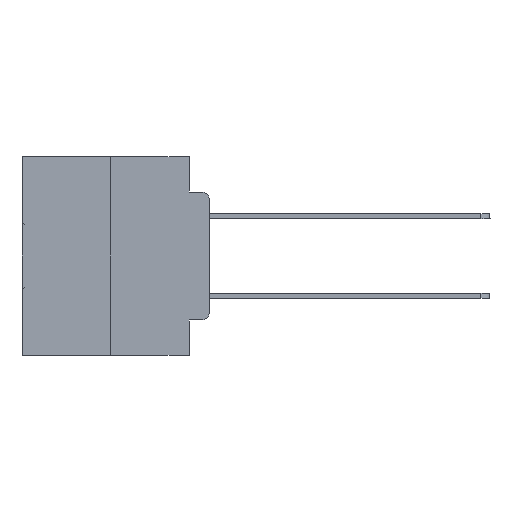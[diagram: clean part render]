
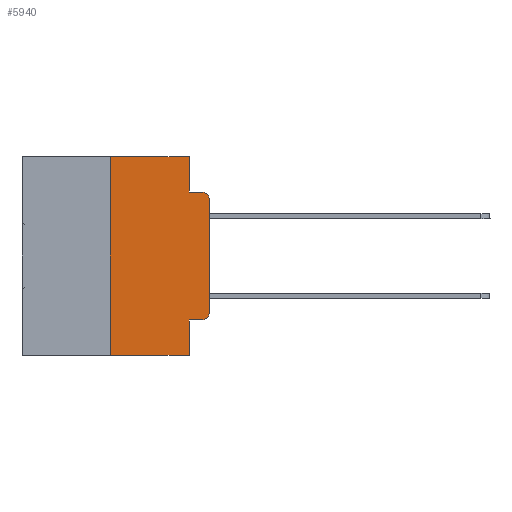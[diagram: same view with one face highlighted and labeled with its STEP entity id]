
A CAD part, left-side view. The second image highlights one B-rep face of the part: STEP entity #5940.
In plain terms, the highlighted planar face has unit normal (-1, 0, 0).
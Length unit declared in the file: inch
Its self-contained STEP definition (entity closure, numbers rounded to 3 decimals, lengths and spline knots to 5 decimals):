
#358 = ORIENTED_EDGE ( 'NONE', *, *, #12259, .T. ) ;
#399 = DIRECTION ( 'NONE',  ( 0., 0., -1. ) ) ;
#882 = VERTEX_POINT ( 'NONE', #4546 ) ;
#1002 = EDGE_LOOP ( 'NONE', ( #21705, #16698, #4040, #10854, #25656, #11242, #358, #7283, #28818, #31168 ) ) ;
#2044 = EDGE_CURVE ( 'NONE', #10015, #7960, #14357, .T. ) ;
#2982 = VECTOR ( 'NONE', #32695, 39.37008 ) ;
#3158 = LINE ( 'NONE', #23463, #16612 ) ;
#3747 = CARTESIAN_POINT ( 'NONE',  ( 0., 0.051, -0.0885 ) ) ;
#3784 = CARTESIAN_POINT ( 'NONE',  ( 0., 0.02, -0.3915 ) ) ;
#3799 = EDGE_CURVE ( 'NONE', #7960, #6192, #8277, .T. ) ;
#4040 = ORIENTED_EDGE ( 'NONE', *, *, #3799, .F. ) ;
#4300 = VERTEX_POINT ( 'NONE', #11045 ) ;
#4436 = EDGE_CURVE ( 'NONE', #30661, #28639, #16899, .T. ) ;
#4546 = CARTESIAN_POINT ( 'NONE',  ( 0., 0., -0.3915 ) ) ;
#4889 = DIRECTION ( 'NONE',  ( -1., 0., 0. ) ) ;
#5033 = CARTESIAN_POINT ( 'NONE',  ( 0., 0.25, 0. ) ) ;
#5524 = EDGE_CURVE ( 'NONE', #4300, #6192, #13404, .T. ) ;
#5940 = ADVANCED_FACE ( 'NONE', ( #27363 ), #13252, .F. ) ;
#6192 = VERTEX_POINT ( 'NONE', #14195 ) ;
#6208 = VERTEX_POINT ( 'NONE', #24257 ) ;
#6360 = DIRECTION ( 'NONE',  ( 0., 0., -1. ) ) ;
#6871 = AXIS2_PLACEMENT_3D ( 'NONE', #19952, #4889, #14978 ) ;
#7283 = ORIENTED_EDGE ( 'NONE', *, *, #4436, .F. ) ;
#7960 = VERTEX_POINT ( 'NONE', #3747 ) ;
#8277 = LINE ( 'NONE', #30936, #14996 ) ;
#8530 = DIRECTION ( 'NONE',  ( 0., -1., 0. ) ) ;
#10015 = VERTEX_POINT ( 'NONE', #29551 ) ;
#10684 = DIRECTION ( 'NONE',  ( 0., 0., -1. ) ) ;
#10854 = ORIENTED_EDGE ( 'NONE', *, *, #2044, .F. ) ;
#11045 = CARTESIAN_POINT ( 'NONE',  ( 0., 0., -0.1085 ) ) ;
#11242 = ORIENTED_EDGE ( 'NONE', *, *, #27987, .F. ) ;
#12259 = EDGE_CURVE ( 'NONE', #6208, #28639, #21976, .T. ) ;
#12766 = CARTESIAN_POINT ( 'NONE',  ( 0., 0., 0. ) ) ;
#12986 = EDGE_CURVE ( 'NONE', #30661, #13514, #32269, .T. ) ;
#13140 = CARTESIAN_POINT ( 'NONE',  ( 0., 0.473, 0. ) ) ;
#13248 = LINE ( 'NONE', #29189, #26452 ) ;
#13252 = PLANE ( 'NONE',  #26390 ) ;
#13404 = CIRCLE ( 'NONE', #6871, 0.02 ) ;
#13480 = EDGE_CURVE ( 'NONE', #16254, #10015, #3158, .T. ) ;
#13514 = VERTEX_POINT ( 'NONE', #23569 ) ;
#13766 = CARTESIAN_POINT ( 'NONE',  ( 0., 0.051, -0.4115 ) ) ;
#14195 = CARTESIAN_POINT ( 'NONE',  ( 0., 0.02, -0.0885 ) ) ;
#14357 = LINE ( 'NONE', #17057, #27572 ) ;
#14978 = DIRECTION ( 'NONE',  ( 0., 0., -1. ) ) ;
#14996 = VECTOR ( 'NONE', #30864, 39.37008 ) ;
#15413 = VECTOR ( 'NONE', #16067, 39.37008 ) ;
#15679 = EDGE_CURVE ( 'NONE', #882, #4300, #29717, .T. ) ;
#15721 = DIRECTION ( 'NONE',  ( 1., 0., 0. ) ) ;
#16067 = DIRECTION ( 'NONE',  ( 0., -1., 0. ) ) ;
#16254 = VERTEX_POINT ( 'NONE', #5033 ) ;
#16612 = VECTOR ( 'NONE', #8530, 39.37008 ) ;
#16698 = ORIENTED_EDGE ( 'NONE', *, *, #5524, .T. ) ;
#16899 = LINE ( 'NONE', #32285, #29806 ) ;
#17057 = CARTESIAN_POINT ( 'NONE',  ( 0., 0.051, 0. ) ) ;
#17272 = DIRECTION ( 'NONE',  ( 0., 0., -1. ) ) ;
#17635 = CARTESIAN_POINT ( 'NONE',  ( 0., 0.051, -0.5 ) ) ;
#19952 = CARTESIAN_POINT ( 'NONE',  ( 0., 0.02, -0.1085 ) ) ;
#21219 = DIRECTION ( 'NONE',  ( 0., -1., 0. ) ) ;
#21364 = DIRECTION ( 'NONE',  ( -1., 0., 0. ) ) ;
#21705 = ORIENTED_EDGE ( 'NONE', *, *, #15679, .T. ) ;
#21976 = LINE ( 'NONE', #30993, #15413 ) ;
#23463 = CARTESIAN_POINT ( 'NONE',  ( 0., 0.473, 0. ) ) ;
#23542 = EDGE_CURVE ( 'NONE', #13514, #882, #30536, .T. ) ;
#23569 = CARTESIAN_POINT ( 'NONE',  ( 0., 0.02, -0.4115 ) ) ;
#24257 = CARTESIAN_POINT ( 'NONE',  ( 0., 0.25, -0.5 ) ) ;
#25602 = VECTOR ( 'NONE', #21219, 39.37008 ) ;
#25656 = ORIENTED_EDGE ( 'NONE', *, *, #13480, .F. ) ;
#26390 = AXIS2_PLACEMENT_3D ( 'NONE', #13140, #15721, #399 ) ;
#26452 = VECTOR ( 'NONE', #31694, 39.37008 ) ;
#27363 = FACE_OUTER_BOUND ( 'NONE', #1002, .T. ) ;
#27572 = VECTOR ( 'NONE', #17272, 39.37008 ) ;
#27987 = EDGE_CURVE ( 'NONE', #6208, #16254, #13248, .T. ) ;
#28083 = CARTESIAN_POINT ( 'NONE',  ( 0., 0.051, -0.4115 ) ) ;
#28639 = VERTEX_POINT ( 'NONE', #17635 ) ;
#28818 = ORIENTED_EDGE ( 'NONE', *, *, #12986, .T. ) ;
#29189 = CARTESIAN_POINT ( 'NONE',  ( 0., 0.25, 0. ) ) ;
#29261 = AXIS2_PLACEMENT_3D ( 'NONE', #3784, #21364, #6360 ) ;
#29551 = CARTESIAN_POINT ( 'NONE',  ( 0., 0.051, 0. ) ) ;
#29717 = LINE ( 'NONE', #12766, #2982 ) ;
#29806 = VECTOR ( 'NONE', #10684, 39.37008 ) ;
#30536 = CIRCLE ( 'NONE', #29261, 0.02 ) ;
#30661 = VERTEX_POINT ( 'NONE', #28083 ) ;
#30864 = DIRECTION ( 'NONE',  ( 0., -1., 0. ) ) ;
#30936 = CARTESIAN_POINT ( 'NONE',  ( 0., 0.051, -0.0885 ) ) ;
#30993 = CARTESIAN_POINT ( 'NONE',  ( 0., 0.473, -0.5 ) ) ;
#31168 = ORIENTED_EDGE ( 'NONE', *, *, #23542, .T. ) ;
#31694 = DIRECTION ( 'NONE',  ( 0., 0., 1. ) ) ;
#32269 = LINE ( 'NONE', #13766, #25602 ) ;
#32285 = CARTESIAN_POINT ( 'NONE',  ( 0., 0.051, 0. ) ) ;
#32695 = DIRECTION ( 'NONE',  ( 0., 0., 1. ) ) ;
